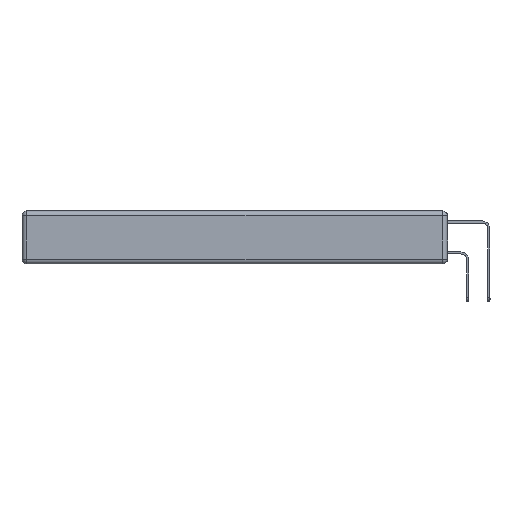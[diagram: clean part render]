
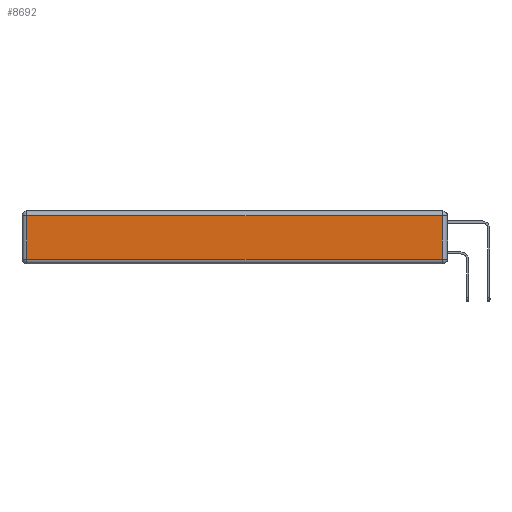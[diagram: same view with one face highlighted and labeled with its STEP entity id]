
A CAD part, left-side view. The second image highlights one B-rep face of the part: STEP entity #8692.
In plain terms, the highlighted planar face has unit normal (-1, 0, 0).
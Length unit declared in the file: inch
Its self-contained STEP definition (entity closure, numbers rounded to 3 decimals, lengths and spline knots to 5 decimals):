
#795 = PLANE ( 'NONE',  #8001 ) ;
#918 = CARTESIAN_POINT ( 'NONE',  ( 0., 0.03, -0.313 ) ) ;
#940 = DIRECTION ( 'NONE',  ( 0., 0., 1. ) ) ;
#1111 = VERTEX_POINT ( 'NONE', #8588 ) ;
#1209 = CARTESIAN_POINT ( 'NONE',  ( 0., 2.72, -0.343 ) ) ;
#1622 = EDGE_CURVE ( 'NONE', #5771, #9984, #9147, .T. ) ;
#1744 = LINE ( 'NONE', #10604, #7266 ) ;
#1887 = DIRECTION ( 'NONE',  ( 0., 0., 1. ) ) ;
#1965 = LINE ( 'NONE', #14583, #2291 ) ;
#2291 = VECTOR ( 'NONE', #1887, 39.37008 ) ;
#2913 = CARTESIAN_POINT ( 'NONE',  ( 0., 2.75, -0.03 ) ) ;
#3945 = ORIENTED_EDGE ( 'NONE', *, *, #9529, .T. ) ;
#4008 = CARTESIAN_POINT ( 'NONE',  ( 0., 2.72, -0.03 ) ) ;
#4260 = CARTESIAN_POINT ( 'NONE',  ( 0., 2.72, -0.313 ) ) ;
#4641 = VERTEX_POINT ( 'NONE', #918 ) ;
#5176 = DIRECTION ( 'NONE',  ( 0., -1., 0. ) ) ;
#5353 = CARTESIAN_POINT ( 'NONE',  ( 0., 0., -0.343 ) ) ;
#5387 = EDGE_CURVE ( 'NONE', #1111, #5771, #9514, .T. ) ;
#5771 = VERTEX_POINT ( 'NONE', #4008 ) ;
#6195 = DIRECTION ( 'NONE',  ( 0., 1., 0. ) ) ;
#6823 = DIRECTION ( 'NONE',  ( 0., 0., -1. ) ) ;
#7266 = VECTOR ( 'NONE', #5176, 39.37008 ) ;
#7553 = VECTOR ( 'NONE', #6823, 39.37008 ) ;
#7556 = EDGE_CURVE ( 'NONE', #9984, #4641, #1744, .T. ) ;
#8001 = AXIS2_PLACEMENT_3D ( 'NONE', #5353, #11201, #940 ) ;
#8588 = CARTESIAN_POINT ( 'NONE',  ( 0., 0.03, -0.03 ) ) ;
#8692 = ADVANCED_FACE ( 'NONE', ( #13518 ), #795, .T. ) ;
#9118 = VECTOR ( 'NONE', #6195, 39.37008 ) ;
#9147 = LINE ( 'NONE', #1209, #7553 ) ;
#9514 = LINE ( 'NONE', #2913, #9118 ) ;
#9529 = EDGE_CURVE ( 'NONE', #4641, #1111, #1965, .T. ) ;
#9984 = VERTEX_POINT ( 'NONE', #4260 ) ;
#10365 = EDGE_LOOP ( 'NONE', ( #12219, #3945, #11944, #12273 ) ) ;
#10604 = CARTESIAN_POINT ( 'NONE',  ( 0., 0., -0.313 ) ) ;
#11201 = DIRECTION ( 'NONE',  ( -1., 0., 0. ) ) ;
#11944 = ORIENTED_EDGE ( 'NONE', *, *, #5387, .T. ) ;
#12219 = ORIENTED_EDGE ( 'NONE', *, *, #7556, .T. ) ;
#12273 = ORIENTED_EDGE ( 'NONE', *, *, #1622, .T. ) ;
#13518 = FACE_OUTER_BOUND ( 'NONE', #10365, .T. ) ;
#14583 = CARTESIAN_POINT ( 'NONE',  ( 0., 0.03, -0.343 ) ) ;
